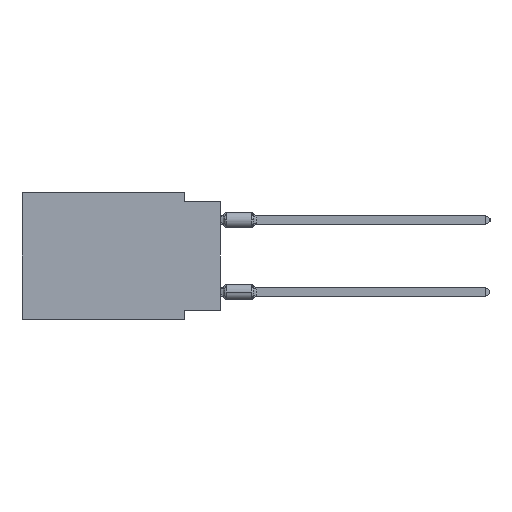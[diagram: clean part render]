
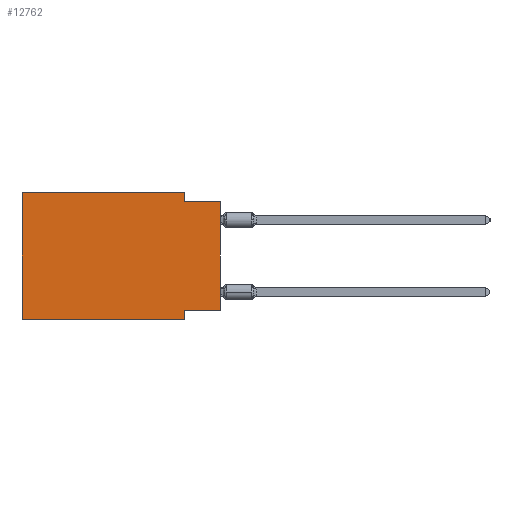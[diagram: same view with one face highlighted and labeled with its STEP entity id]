
A CAD part, left-side view. The second image highlights one B-rep face of the part: STEP entity #12762.
In plain terms, the highlighted planar face has unit normal (-1, 0, 0).
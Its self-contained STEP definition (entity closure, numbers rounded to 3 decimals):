
#831 = CARTESIAN_POINT ( 'NONE',  ( 0., 13.97, 0. ) ) ;
#1688 = VERTEX_POINT ( 'NONE', #39973 ) ;
#2051 = LINE ( 'NONE', #36334, #2465 ) ;
#2465 = VECTOR ( 'NONE', #35222, 1000. ) ;
#2527 = VERTEX_POINT ( 'NONE', #37271 ) ;
#2804 = LINE ( 'NONE', #28778, #4168 ) ;
#2922 = CARTESIAN_POINT ( 'NONE',  ( 0., 13.97, 0. ) ) ;
#4168 = VECTOR ( 'NONE', #7508, 1000. ) ;
#4474 = CARTESIAN_POINT ( 'NONE',  ( 0., 2.54, 0. ) ) ;
#5634 = EDGE_CURVE ( 'NONE', #11240, #45020, #27958, .T. ) ;
#7343 = DIRECTION ( 'NONE',  ( 0., 0., -1. ) ) ;
#7392 = CARTESIAN_POINT ( 'NONE',  ( 0., 2.54, -0.635 ) ) ;
#7508 = DIRECTION ( 'NONE',  ( 0., -1., 0. ) ) ;
#7603 = CARTESIAN_POINT ( 'NONE',  ( 0., 0., -0.635 ) ) ;
#11240 = VERTEX_POINT ( 'NONE', #52412 ) ;
#11468 = VECTOR ( 'NONE', #37179, 1000. ) ;
#12762 = ADVANCED_FACE ( 'NONE', ( #45225 ), #28070, .F. ) ;
#13379 = VERTEX_POINT ( 'NONE', #4474 ) ;
#13834 = VECTOR ( 'NONE', #16079, 1000. ) ;
#14856 = EDGE_CURVE ( 'NONE', #1688, #11240, #16867, .T. ) ;
#15040 = ORIENTED_EDGE ( 'NONE', *, *, #48656, .F. ) ;
#15241 = LINE ( 'NONE', #40956, #13834 ) ;
#15537 = DIRECTION ( 'NONE',  ( 0., 0., -1. ) ) ;
#16079 = DIRECTION ( 'NONE',  ( 0., 0., -1. ) ) ;
#16867 = LINE ( 'NONE', #33710, #48962 ) ;
#17962 = EDGE_CURVE ( 'NONE', #13379, #23076, #15241, .T. ) ;
#17979 = EDGE_CURVE ( 'NONE', #2527, #45020, #2804, .T. ) ;
#19731 = EDGE_LOOP ( 'NONE', ( #39720, #15040, #32642, #48969, #35769, #31535, #39316, #39441 ) ) ;
#20746 = DIRECTION ( 'NONE',  ( 0., 1., 0. ) ) ;
#23076 = VERTEX_POINT ( 'NONE', #7392 ) ;
#24806 = DIRECTION ( 'NONE',  ( 0., 0., 1. ) ) ;
#27375 = EDGE_CURVE ( 'NONE', #2527, #29234, #2051, .T. ) ;
#27682 = CARTESIAN_POINT ( 'NONE',  ( 0., 2.54, -8.89 ) ) ;
#27713 = CARTESIAN_POINT ( 'NONE',  ( 0., 0., -0.635 ) ) ;
#27742 = VECTOR ( 'NONE', #32964, 1000. ) ;
#27958 = LINE ( 'NONE', #27682, #50874 ) ;
#28070 = PLANE ( 'NONE',  #31242 ) ;
#28778 = CARTESIAN_POINT ( 'NONE',  ( 0., 13.97, -8.89 ) ) ;
#29234 = VERTEX_POINT ( 'NONE', #831 ) ;
#31242 = AXIS2_PLACEMENT_3D ( 'NONE', #2922, #45504, #7343 ) ;
#31535 = ORIENTED_EDGE ( 'NONE', *, *, #17979, .T. ) ;
#32642 = ORIENTED_EDGE ( 'NONE', *, *, #17962, .F. ) ;
#32838 = CARTESIAN_POINT ( 'NONE',  ( 0., 0., 0. ) ) ;
#32964 = DIRECTION ( 'NONE',  ( 0., -1., 0. ) ) ;
#33710 = CARTESIAN_POINT ( 'NONE',  ( 0., 0., -8.255 ) ) ;
#34660 = VECTOR ( 'NONE', #24806, 1000. ) ;
#35222 = DIRECTION ( 'NONE',  ( 0., 0., 1. ) ) ;
#35769 = ORIENTED_EDGE ( 'NONE', *, *, #27375, .F. ) ;
#36334 = CARTESIAN_POINT ( 'NONE',  ( 0., 13.97, 0. ) ) ;
#37179 = DIRECTION ( 'NONE',  ( 0., -1., 0. ) ) ;
#37271 = CARTESIAN_POINT ( 'NONE',  ( 0., 13.97, -8.89 ) ) ;
#39316 = ORIENTED_EDGE ( 'NONE', *, *, #5634, .F. ) ;
#39441 = ORIENTED_EDGE ( 'NONE', *, *, #14856, .F. ) ;
#39720 = ORIENTED_EDGE ( 'NONE', *, *, #51134, .T. ) ;
#39973 = CARTESIAN_POINT ( 'NONE',  ( 0., 0., -8.255 ) ) ;
#40956 = CARTESIAN_POINT ( 'NONE',  ( 0., 2.54, 0. ) ) ;
#41276 = LINE ( 'NONE', #42081, #27742 ) ;
#41411 = CARTESIAN_POINT ( 'NONE',  ( 0., 2.54, -8.89 ) ) ;
#42081 = CARTESIAN_POINT ( 'NONE',  ( 0., 13.97, 0. ) ) ;
#42332 = VERTEX_POINT ( 'NONE', #27713 ) ;
#45020 = VERTEX_POINT ( 'NONE', #41411 ) ;
#45225 = FACE_OUTER_BOUND ( 'NONE', #19731, .T. ) ;
#45489 = LINE ( 'NONE', #7603, #11468 ) ;
#45504 = DIRECTION ( 'NONE',  ( 1., 0., 0. ) ) ;
#48656 = EDGE_CURVE ( 'NONE', #23076, #42332, #45489, .T. ) ;
#48962 = VECTOR ( 'NONE', #20746, 1000. ) ;
#48969 = ORIENTED_EDGE ( 'NONE', *, *, #53108, .F. ) ;
#50874 = VECTOR ( 'NONE', #15537, 1000. ) ;
#51134 = EDGE_CURVE ( 'NONE', #1688, #42332, #53594, .T. ) ;
#52412 = CARTESIAN_POINT ( 'NONE',  ( 0., 2.54, -8.255 ) ) ;
#53108 = EDGE_CURVE ( 'NONE', #29234, #13379, #41276, .T. ) ;
#53594 = LINE ( 'NONE', #32838, #34660 ) ;
